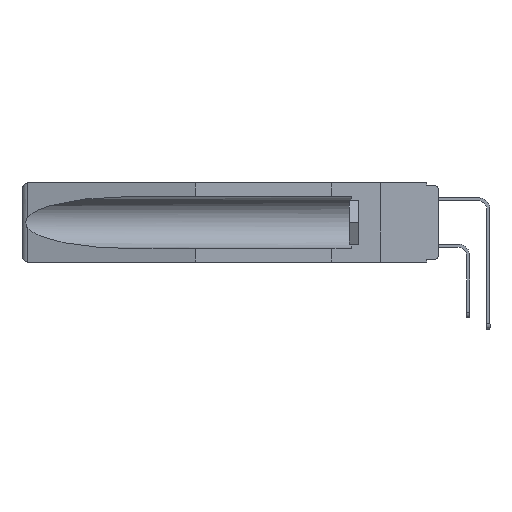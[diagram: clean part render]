
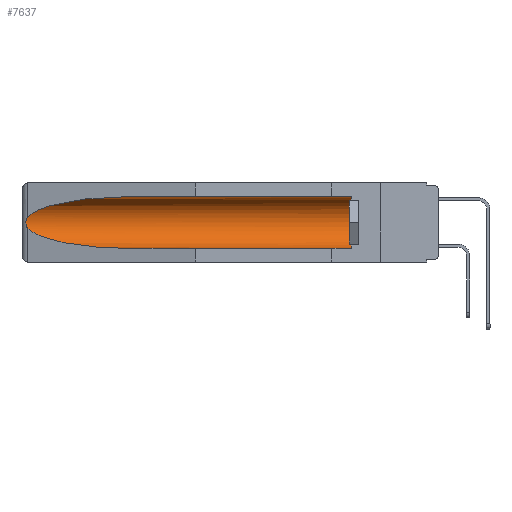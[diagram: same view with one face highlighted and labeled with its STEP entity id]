
A CAD part, left-side view. The second image highlights one B-rep face of the part: STEP entity #7637.
In plain terms, the highlighted cylindrical face has radius 2.857 mm (diameter 5.715 mm), a partial arc.
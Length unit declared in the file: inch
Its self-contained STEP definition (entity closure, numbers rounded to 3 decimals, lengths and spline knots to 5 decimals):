
#571 = CARTESIAN_POINT ( 'NONE',  ( 0.155, 0.126, -0.284 ) ) ;
#1200 = CARTESIAN_POINT ( 'NONE',  ( 0.155, 0.126, -0.1715 ) ) ;
#1369 = CARTESIAN_POINT ( 'NONE',  ( 0.26537, 1.52718, -0.19328 ) ) ;
#2348 = AXIS2_PLACEMENT_3D ( 'NONE', #1200, #16574, #17955 ) ;
#2400 = CARTESIAN_POINT ( 'NONE',  ( 0.26537, 1.52718, -0.19328 ) ) ;
#2793 = EDGE_CURVE ( 'NONE', #13065, #11160, #9337, .T. ) ;
#3030 = CARTESIAN_POINT ( 'NONE',  ( 0.21114, 1.30732, -0.059 ) ) ;
#3296 = VERTEX_POINT ( 'NONE', #6687 ) ;
#3358 = DIRECTION ( 'NONE',  ( 0., 1., 0. ) ) ;
#4002 = EDGE_CURVE ( 'NONE', #7028, #9115, #14174, .T. ) ;
#4160 = CARTESIAN_POINT ( 'NONE',  ( 0.155, 1.07973, -0.059 ) ) ;
#5423 = CARTESIAN_POINT ( 'NONE',  ( 0.155, -0.30754, -0.284 ) ) ;
#5483 = EDGE_LOOP ( 'NONE', ( #13728, #10508, #14702, #11269, #12077, #16906 ) ) ;
#6234 = LINE ( 'NONE', #7700, #11122 ) ;
#6455 = CARTESIAN_POINT ( 'NONE',  ( 0.155, 0.126, -0.059 ) ) ;
#6630 = CARTESIAN_POINT ( 'NONE',  ( 0.155, -0.30754, -0.1715 ) ) ;
#6649 = CARTESIAN_POINT ( 'NONE',  ( 0.26597, 1.52961, -0.15275 ) ) ;
#6687 = CARTESIAN_POINT ( 'NONE',  ( 0.26537, 1.52718, -0.14972 ) ) ;
#6888 = DIRECTION ( 'NONE',  ( 0., 1., 0. ) ) ;
#7028 = VERTEX_POINT ( 'NONE', #571 ) ;
#7076 = CARTESIAN_POINT ( 'NONE',  ( 0.155, 1.07973, -0.284 ) ) ;
#7217 = EDGE_CURVE ( 'NONE', #3296, #13065, #12785, .T. ) ;
#7409 = VERTEX_POINT ( 'NONE', #4160 ) ;
#7637 = ADVANCED_FACE ( 'NONE', ( #13569 ), #8105, .F. ) ;
#7700 = CARTESIAN_POINT ( 'NONE',  ( 0.155, -0.30754, -0.059 ) ) ;
#7829 = DIRECTION ( 'NONE',  ( 0., 0., 1. ) ) ;
#7948 = CARTESIAN_POINT ( 'NONE',  ( 0.26537, 1.52718, -0.14972 ) ) ;
#8105 = CYLINDRICAL_SURFACE ( 'NONE', #10530, 0.1125 ) ;
#8272 = LINE ( 'NONE', #5423, #12823 ) ;
#9115 = VERTEX_POINT ( 'NONE', #6455 ) ;
#9337 =( BOUNDED_CURVE ( )  B_SPLINE_CURVE ( 3, ( #14200, #15507, #14110, #7076 ),
 .UNSPECIFIED., .F., .T. ) 
 B_SPLINE_CURVE_WITH_KNOTS ( ( 4, 4 ),
 ( 0.1948, 1.5708 ),
 .UNSPECIFIED. ) 
 CURVE ( )  GEOMETRIC_REPRESENTATION_ITEM ( )  RATIONAL_B_SPLINE_CURVE ( ( 1., 0.848, 0.848, 1. ) ) 
 REPRESENTATION_ITEM ( '' )  );
#9513 = CARTESIAN_POINT ( 'NONE',  ( 0.2673, 1.53269, -0.17917 ) ) ;
#9564 = EDGE_CURVE ( 'NONE', #7028, #11160, #8272, .T. ) ;
#9828 =( BOUNDED_CURVE ( )  B_SPLINE_CURVE ( 3, ( #17206, #3030, #13204, #14590 ),
 .UNSPECIFIED., .F., .F. ) 
 B_SPLINE_CURVE_WITH_KNOTS ( ( 4, 4 ),
 ( 4.71239, 6.08839 ),
 .UNSPECIFIED. ) 
 CURVE ( )  GEOMETRIC_REPRESENTATION_ITEM ( )  RATIONAL_B_SPLINE_CURVE ( ( 1., 0.848, 0.848, 1. ) ) 
 REPRESENTATION_ITEM ( '' )  );
#10508 = ORIENTED_EDGE ( 'NONE', *, *, #7217, .T. ) ;
#10530 = AXIS2_PLACEMENT_3D ( 'NONE', #6630, #17940, #7829 ) ;
#10896 = CARTESIAN_POINT ( 'NONE',  ( 0.2675, 1.53308, -0.16763 ) ) ;
#10988 = CARTESIAN_POINT ( 'NONE',  ( 0.2675, 1.53308, -0.17534 ) ) ;
#11122 = VECTOR ( 'NONE', #3358, 39.37008 ) ;
#11160 = VERTEX_POINT ( 'NONE', #13235 ) ;
#11269 = ORIENTED_EDGE ( 'NONE', *, *, #9564, .F. ) ;
#12077 = ORIENTED_EDGE ( 'NONE', *, *, #4002, .T. ) ;
#12102 = CARTESIAN_POINT ( 'NONE',  ( 0.26597, 1.5296, -0.19026 ) ) ;
#12278 = CARTESIAN_POINT ( 'NONE',  ( 0.26655, 1.53094, -0.18657 ) ) ;
#12785 = B_SPLINE_CURVE_WITH_KNOTS ( 'NONE', 3,
 ( #7948, #6649, #16672, #13496, #10896, #10988, #9513, #12278, #12102, #2400 ),
 .UNSPECIFIED., .F., .F.,
 ( 4, 2, 2, 2, 4 ),
 ( 0., 0.00029, 0.00058, 0.00087, 0.00117 ),
 .UNSPECIFIED. ) ;
#12823 = VECTOR ( 'NONE', #6888, 39.37008 ) ;
#13065 = VERTEX_POINT ( 'NONE', #1369 ) ;
#13204 = CARTESIAN_POINT ( 'NONE',  ( 0.25451, 1.48313, -0.09465 ) ) ;
#13235 = CARTESIAN_POINT ( 'NONE',  ( 0.155, 1.07973, -0.284 ) ) ;
#13496 = CARTESIAN_POINT ( 'NONE',  ( 0.2673, 1.5327, -0.16383 ) ) ;
#13569 = FACE_OUTER_BOUND ( 'NONE', #5483, .T. ) ;
#13728 = ORIENTED_EDGE ( 'NONE', *, *, #16664, .T. ) ;
#13807 = EDGE_CURVE ( 'NONE', #9115, #7409, #6234, .T. ) ;
#14110 = CARTESIAN_POINT ( 'NONE',  ( 0.21114, 1.30732, -0.284 ) ) ;
#14174 = CIRCLE ( 'NONE', #2348, 0.1125 ) ;
#14200 = CARTESIAN_POINT ( 'NONE',  ( 0.26537, 1.52718, -0.19328 ) ) ;
#14590 = CARTESIAN_POINT ( 'NONE',  ( 0.26537, 1.52718, -0.14972 ) ) ;
#14702 = ORIENTED_EDGE ( 'NONE', *, *, #2793, .T. ) ;
#15507 = CARTESIAN_POINT ( 'NONE',  ( 0.25451, 1.48313, -0.24835 ) ) ;
#16574 = DIRECTION ( 'NONE',  ( 0., -1., 0. ) ) ;
#16664 = EDGE_CURVE ( 'NONE', #7409, #3296, #9828, .T. ) ;
#16672 = CARTESIAN_POINT ( 'NONE',  ( 0.26654, 1.53092, -0.15636 ) ) ;
#16906 = ORIENTED_EDGE ( 'NONE', *, *, #13807, .T. ) ;
#17206 = CARTESIAN_POINT ( 'NONE',  ( 0.155, 1.07973, -0.059 ) ) ;
#17940 = DIRECTION ( 'NONE',  ( 0., 1., 0. ) ) ;
#17955 = DIRECTION ( 'NONE',  ( 0., 0., 1. ) ) ;
